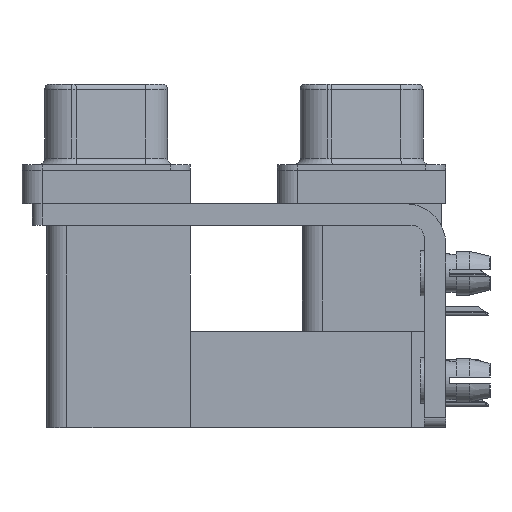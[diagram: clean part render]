
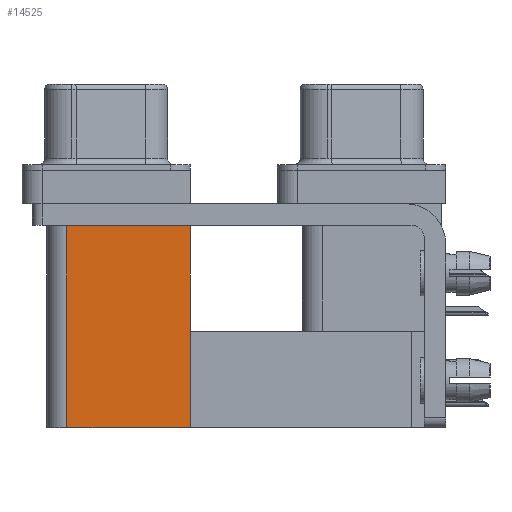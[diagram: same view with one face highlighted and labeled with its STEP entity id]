
A CAD part, left-side view. The second image highlights one B-rep face of the part: STEP entity #14525.
In plain terms, the highlighted planar face has unit normal (-1, 0, 0).
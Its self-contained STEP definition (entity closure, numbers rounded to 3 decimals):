
#947 = PLANE ( 'NONE',  #33780 ) ;
#3738 = CARTESIAN_POINT ( 'NONE',  ( 3.7, 21.975, -2.5 ) ) ;
#4001 = VERTEX_POINT ( 'NONE', #9397 ) ;
#7104 = DIRECTION ( 'NONE',  ( 0., 1., 0. ) ) ;
#7319 = DIRECTION ( 'NONE',  ( 1., 0., 0. ) ) ;
#9397 = CARTESIAN_POINT ( 'NONE',  ( 3.7, 12.775, -19.2 ) ) ;
#10388 = ORIENTED_EDGE ( 'NONE', *, *, #32362, .F. ) ;
#11607 = VERTEX_POINT ( 'NONE', #27878 ) ;
#11806 = DIRECTION ( 'NONE',  ( 0., 1., 0. ) ) ;
#11973 = VECTOR ( 'NONE', #11806, 1000. ) ;
#12486 = DIRECTION ( 'NONE',  ( 0., 0., 1. ) ) ;
#12857 = LINE ( 'NONE', #16648, #16066 ) ;
#13267 = DIRECTION ( 'NONE',  ( 0., 0., 1. ) ) ;
#13614 = VECTOR ( 'NONE', #16556, 1000. ) ;
#14525 = ADVANCED_FACE ( 'NONE', ( #16276 ), #947, .F. ) ;
#16066 = VECTOR ( 'NONE', #13267, 1000. ) ;
#16276 = FACE_OUTER_BOUND ( 'NONE', #38986, .T. ) ;
#16367 = CARTESIAN_POINT ( 'NONE',  ( 3.7, 12.775, -2.5 ) ) ;
#16556 = DIRECTION ( 'NONE',  ( 0., 1., 0. ) ) ;
#16648 = CARTESIAN_POINT ( 'NONE',  ( 3.7, 21.975, -19.2 ) ) ;
#17626 = EDGE_CURVE ( 'NONE', #11607, #38049, #32094, .T. ) ;
#18126 = ORIENTED_EDGE ( 'NONE', *, *, #32588, .F. ) ;
#18733 = VERTEX_POINT ( 'NONE', #31521 ) ;
#20767 = VECTOR ( 'NONE', #12486, 1000. ) ;
#21419 = CARTESIAN_POINT ( 'NONE',  ( 3.7, 12.775, -19.2 ) ) ;
#21580 = CARTESIAN_POINT ( 'NONE',  ( 3.7, 12.775, -19.2 ) ) ;
#23072 = CARTESIAN_POINT ( 'NONE',  ( 3.7, 12.775, -19.2 ) ) ;
#24297 = ORIENTED_EDGE ( 'NONE', *, *, #17626, .T. ) ;
#25282 = ORIENTED_EDGE ( 'NONE', *, *, #31928, .T. ) ;
#27878 = CARTESIAN_POINT ( 'NONE',  ( 3.7, 12.775, -2.5 ) ) ;
#31369 = LINE ( 'NONE', #21580, #11973 ) ;
#31521 = CARTESIAN_POINT ( 'NONE',  ( 3.7, 21.975, -19.2 ) ) ;
#31928 = EDGE_CURVE ( 'NONE', #4001, #11607, #37610, .T. ) ;
#32094 = LINE ( 'NONE', #16367, #13614 ) ;
#32362 = EDGE_CURVE ( 'NONE', #4001, #18733, #31369, .T. ) ;
#32588 = EDGE_CURVE ( 'NONE', #18733, #38049, #12857, .T. ) ;
#33780 = AXIS2_PLACEMENT_3D ( 'NONE', #23072, #7319, #7104 ) ;
#37610 = LINE ( 'NONE', #21419, #20767 ) ;
#38049 = VERTEX_POINT ( 'NONE', #3738 ) ;
#38986 = EDGE_LOOP ( 'NONE', ( #24297, #18126, #10388, #25282 ) ) ;
